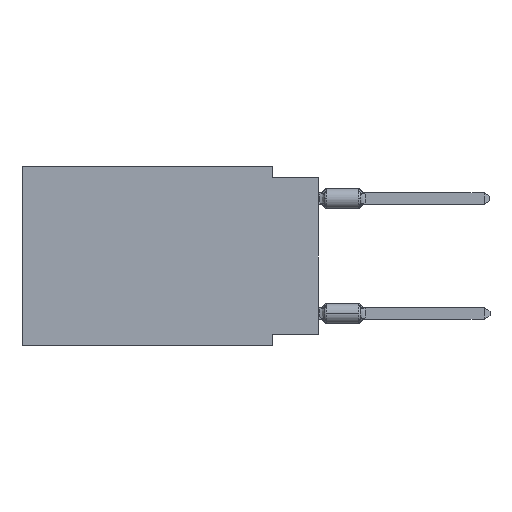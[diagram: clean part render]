
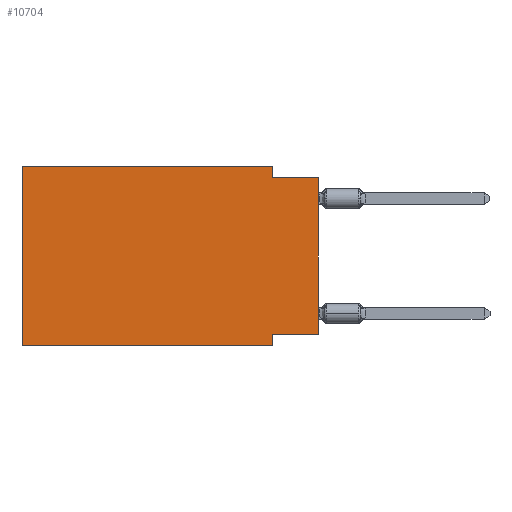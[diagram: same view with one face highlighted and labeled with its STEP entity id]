
A CAD part, left-side view. The second image highlights one B-rep face of the part: STEP entity #10704.
In plain terms, the highlighted planar face has unit normal (-1, 0, 0).
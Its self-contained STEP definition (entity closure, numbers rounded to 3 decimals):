
#122 = ORIENTED_EDGE ( 'NONE', *, *, #13427, .F. ) ;
#488 = ORIENTED_EDGE ( 'NONE', *, *, #18106, .F. ) ;
#921 = LINE ( 'NONE', #14769, #13061 ) ;
#1335 = DIRECTION ( 'NONE',  ( 0., -1., 0. ) ) ;
#1797 = LINE ( 'NONE', #5798, #6023 ) ;
#1855 = CARTESIAN_POINT ( 'NONE',  ( 0., 2.54, 0. ) ) ;
#2511 = DIRECTION ( 'NONE',  ( 0., 0., -1. ) ) ;
#2876 = VECTOR ( 'NONE', #9741, 1000. ) ;
#2915 = VERTEX_POINT ( 'NONE', #13231 ) ;
#3117 = DIRECTION ( 'NONE',  ( 0., -1., 0. ) ) ;
#3324 = EDGE_CURVE ( 'NONE', #8351, #6572, #7597, .T. ) ;
#3836 = CARTESIAN_POINT ( 'NONE',  ( 0., 2.54, -9.271 ) ) ;
#4309 = FACE_OUTER_BOUND ( 'NONE', #24994, .T. ) ;
#5100 = VERTEX_POINT ( 'NONE', #18452 ) ;
#5746 = EDGE_CURVE ( 'NONE', #13038, #5100, #16724, .T. ) ;
#5798 = CARTESIAN_POINT ( 'NONE',  ( 0., 0., -9.271 ) ) ;
#6023 = VECTOR ( 'NONE', #11239, 1000. ) ;
#6195 = ORIENTED_EDGE ( 'NONE', *, *, #22962, .T. ) ;
#6218 = EDGE_CURVE ( 'NONE', #15675, #8351, #1797, .T. ) ;
#6368 = PLANE ( 'NONE',  #18655 ) ;
#6572 = VERTEX_POINT ( 'NONE', #23903 ) ;
#7246 = CARTESIAN_POINT ( 'NONE',  ( 0., 0., -0.635 ) ) ;
#7319 = ORIENTED_EDGE ( 'NONE', *, *, #10768, .T. ) ;
#7399 = CARTESIAN_POINT ( 'NONE',  ( 0., 16.383, -9.906 ) ) ;
#7583 = ORIENTED_EDGE ( 'NONE', *, *, #5746, .F. ) ;
#7597 = LINE ( 'NONE', #11998, #14957 ) ;
#7930 = LINE ( 'NONE', #1855, #2876 ) ;
#8351 = VERTEX_POINT ( 'NONE', #3836 ) ;
#8595 = DIRECTION ( 'NONE',  ( 0., 0., 1. ) ) ;
#9099 = DIRECTION ( 'NONE',  ( 0., 0., 1. ) ) ;
#9116 = VERTEX_POINT ( 'NONE', #15408 ) ;
#9366 = ORIENTED_EDGE ( 'NONE', *, *, #3324, .F. ) ;
#9741 = DIRECTION ( 'NONE',  ( 0., 0., -1. ) ) ;
#10659 = LINE ( 'NONE', #18706, #18081 ) ;
#10704 = ADVANCED_FACE ( 'NONE', ( #4309 ), #6368, .F. ) ;
#10743 = VECTOR ( 'NONE', #9099, 1000. ) ;
#10761 = CARTESIAN_POINT ( 'NONE',  ( 0., 16.383, 0. ) ) ;
#10768 = EDGE_CURVE ( 'NONE', #2915, #6572, #22948, .T. ) ;
#11208 = VECTOR ( 'NONE', #1335, 1000. ) ;
#11239 = DIRECTION ( 'NONE',  ( 0., 1., 0. ) ) ;
#11557 = LINE ( 'NONE', #24908, #10743 ) ;
#11928 = CARTESIAN_POINT ( 'NONE',  ( 0., 0., -9.271 ) ) ;
#11998 = CARTESIAN_POINT ( 'NONE',  ( 0., 2.54, -9.906 ) ) ;
#13038 = VERTEX_POINT ( 'NONE', #20308 ) ;
#13061 = VECTOR ( 'NONE', #16337, 1000. ) ;
#13198 = EDGE_CURVE ( 'NONE', #2915, #19955, #11557, .T. ) ;
#13231 = CARTESIAN_POINT ( 'NONE',  ( 0., 16.383, -9.906 ) ) ;
#13427 = EDGE_CURVE ( 'NONE', #9116, #13038, #7930, .T. ) ;
#13945 = DIRECTION ( 'NONE',  ( 0., 0., -1. ) ) ;
#14283 = CARTESIAN_POINT ( 'NONE',  ( 0., 16.383, 0. ) ) ;
#14769 = CARTESIAN_POINT ( 'NONE',  ( 0., 16.383, 0. ) ) ;
#14957 = VECTOR ( 'NONE', #13945, 1000. ) ;
#15408 = CARTESIAN_POINT ( 'NONE',  ( 0., 2.54, 0. ) ) ;
#15675 = VERTEX_POINT ( 'NONE', #11928 ) ;
#16337 = DIRECTION ( 'NONE',  ( 0., -1., 0. ) ) ;
#16724 = LINE ( 'NONE', #7246, #25033 ) ;
#18081 = VECTOR ( 'NONE', #8595, 1000. ) ;
#18106 = EDGE_CURVE ( 'NONE', #19955, #9116, #921, .T. ) ;
#18452 = CARTESIAN_POINT ( 'NONE',  ( 0., 0., -0.635 ) ) ;
#18655 = AXIS2_PLACEMENT_3D ( 'NONE', #14283, #22200, #2511 ) ;
#18706 = CARTESIAN_POINT ( 'NONE',  ( 0., 0., 0. ) ) ;
#19955 = VERTEX_POINT ( 'NONE', #10761 ) ;
#20308 = CARTESIAN_POINT ( 'NONE',  ( 0., 2.54, -0.635 ) ) ;
#21965 = ORIENTED_EDGE ( 'NONE', *, *, #6218, .F. ) ;
#22200 = DIRECTION ( 'NONE',  ( 1., 0., 0. ) ) ;
#22506 = ORIENTED_EDGE ( 'NONE', *, *, #13198, .F. ) ;
#22948 = LINE ( 'NONE', #7399, #11208 ) ;
#22962 = EDGE_CURVE ( 'NONE', #15675, #5100, #10659, .T. ) ;
#23903 = CARTESIAN_POINT ( 'NONE',  ( 0., 2.54, -9.906 ) ) ;
#24908 = CARTESIAN_POINT ( 'NONE',  ( 0., 16.383, 0. ) ) ;
#24994 = EDGE_LOOP ( 'NONE', ( #6195, #7583, #122, #488, #22506, #7319, #9366, #21965 ) ) ;
#25033 = VECTOR ( 'NONE', #3117, 1000. ) ;
